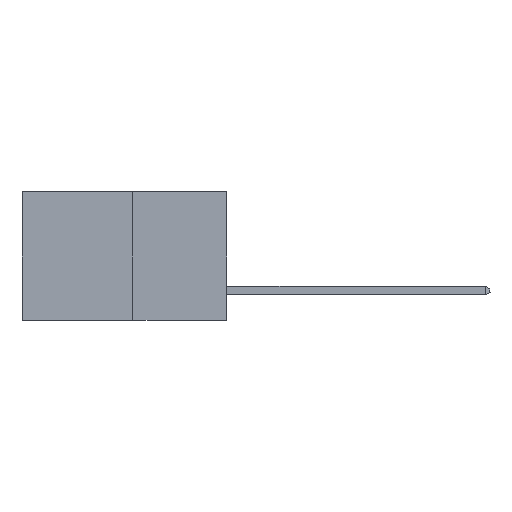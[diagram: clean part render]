
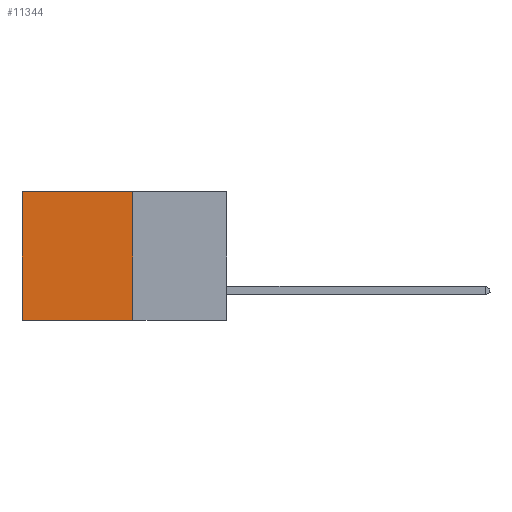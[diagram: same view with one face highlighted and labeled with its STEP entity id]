
A CAD part, left-side view. The second image highlights one B-rep face of the part: STEP entity #11344.
In plain terms, the highlighted planar face has unit normal (-1, 0, 0).
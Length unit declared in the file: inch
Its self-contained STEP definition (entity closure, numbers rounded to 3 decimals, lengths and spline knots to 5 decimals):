
#126 = CARTESIAN_POINT ( 'NONE',  ( 0.277, 0.27, 0. ) ) ;
#586 = CARTESIAN_POINT ( 'NONE',  ( 0.277, 0.27, 0. ) ) ;
#598 = DIRECTION ( 'NONE',  ( 0., 0., -1. ) ) ;
#1586 = CARTESIAN_POINT ( 'NONE',  ( 0.277, 0.27, -0.37 ) ) ;
#2117 = EDGE_CURVE ( 'NONE', #7148, #8496, #7534, .T. ) ;
#2558 = VECTOR ( 'NONE', #9428, 39.37008 ) ;
#2792 = EDGE_CURVE ( 'NONE', #5772, #4765, #13583, .T. ) ;
#2832 = ORIENTED_EDGE ( 'NONE', *, *, #9657, .T. ) ;
#3250 = EDGE_CURVE ( 'NONE', #5772, #7148, #11191, .T. ) ;
#3916 = DIRECTION ( 'NONE',  ( 0., 0., -1. ) ) ;
#4729 = VECTOR ( 'NONE', #12592, 39.37008 ) ;
#4765 = VERTEX_POINT ( 'NONE', #11452 ) ;
#5111 = PLANE ( 'NONE',  #6418 ) ;
#5506 = VECTOR ( 'NONE', #13439, 39.37008 ) ;
#5772 = VERTEX_POINT ( 'NONE', #126 ) ;
#5925 = CARTESIAN_POINT ( 'NONE',  ( 0.277, 0.27, -0.37 ) ) ;
#5980 = LINE ( 'NONE', #11352, #8527 ) ;
#6418 = AXIS2_PLACEMENT_3D ( 'NONE', #13260, #7230, #598 ) ;
#6627 = FACE_OUTER_BOUND ( 'NONE', #10565, .T. ) ;
#6707 = ORIENTED_EDGE ( 'NONE', *, *, #2117, .F. ) ;
#7148 = VERTEX_POINT ( 'NONE', #1586 ) ;
#7230 = DIRECTION ( 'NONE',  ( 1., 0., 0. ) ) ;
#7534 = LINE ( 'NONE', #5925, #4729 ) ;
#8496 = VERTEX_POINT ( 'NONE', #12251 ) ;
#8527 = VECTOR ( 'NONE', #3916, 39.37008 ) ;
#9428 = DIRECTION ( 'NONE',  ( 0., 0., -1. ) ) ;
#9540 = CARTESIAN_POINT ( 'NONE',  ( 0.277, 0.27, -0.37 ) ) ;
#9657 = EDGE_CURVE ( 'NONE', #4765, #8496, #5980, .T. ) ;
#9870 = ORIENTED_EDGE ( 'NONE', *, *, #2792, .T. ) ;
#10565 = EDGE_LOOP ( 'NONE', ( #2832, #6707, #12839, #9870 ) ) ;
#11191 = LINE ( 'NONE', #9540, #2558 ) ;
#11344 = ADVANCED_FACE ( 'NONE', ( #6627 ), #5111, .F. ) ;
#11352 = CARTESIAN_POINT ( 'NONE',  ( 0.277, 0.59, -0.37 ) ) ;
#11452 = CARTESIAN_POINT ( 'NONE',  ( 0.277, 0.59, 0. ) ) ;
#12251 = CARTESIAN_POINT ( 'NONE',  ( 0.277, 0.59, -0.37 ) ) ;
#12592 = DIRECTION ( 'NONE',  ( 0., 1., 0. ) ) ;
#12839 = ORIENTED_EDGE ( 'NONE', *, *, #3250, .F. ) ;
#13260 = CARTESIAN_POINT ( 'NONE',  ( 0.277, 0.27, -0.37 ) ) ;
#13439 = DIRECTION ( 'NONE',  ( 0., 1., 0. ) ) ;
#13583 = LINE ( 'NONE', #586, #5506 ) ;
